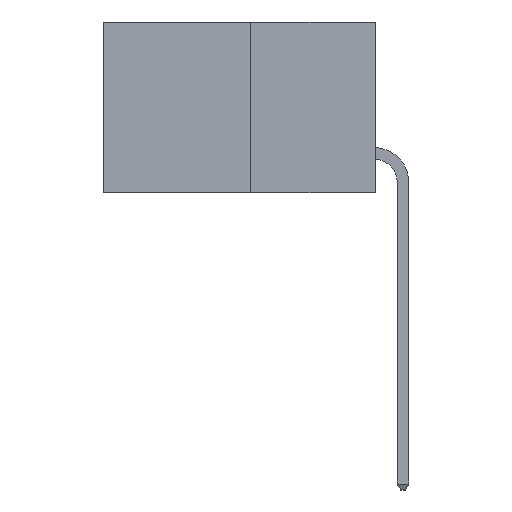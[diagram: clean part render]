
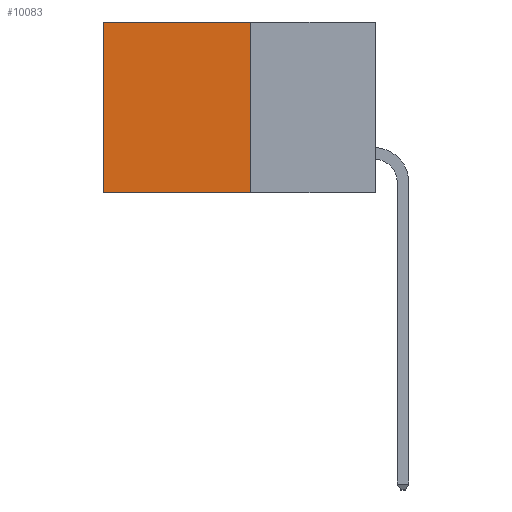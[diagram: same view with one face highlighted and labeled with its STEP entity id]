
A CAD part, left-side view. The second image highlights one B-rep face of the part: STEP entity #10083.
In plain terms, the highlighted planar face has unit normal (-1, 0, 0).
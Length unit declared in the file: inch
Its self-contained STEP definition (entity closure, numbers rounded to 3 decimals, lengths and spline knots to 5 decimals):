
#77 = CARTESIAN_POINT ( 'NONE',  ( 0.277, 0.27, -0.37 ) ) ;
#220 = VECTOR ( 'NONE', #15139, 39.37008 ) ;
#687 = LINE ( 'NONE', #77, #1678 ) ;
#996 = DIRECTION ( 'NONE',  ( 0., 1., 0. ) ) ;
#1178 = DIRECTION ( 'NONE',  ( 1., 0., 0. ) ) ;
#1315 = CARTESIAN_POINT ( 'NONE',  ( 0.277, 0.27, -0.37 ) ) ;
#1673 = DIRECTION ( 'NONE',  ( 0., 0., -1. ) ) ;
#1678 = VECTOR ( 'NONE', #1673, 39.37008 ) ;
#2572 = CARTESIAN_POINT ( 'NONE',  ( 0.277, 0.27, -0.37 ) ) ;
#3285 = VERTEX_POINT ( 'NONE', #3887 ) ;
#3887 = CARTESIAN_POINT ( 'NONE',  ( 0.277, 0.27, 0. ) ) ;
#4393 = CARTESIAN_POINT ( 'NONE',  ( 0.277, 0.27, 0. ) ) ;
#4779 = AXIS2_PLACEMENT_3D ( 'NONE', #8943, #1178, #11983 ) ;
#5387 = VERTEX_POINT ( 'NONE', #1315 ) ;
#6457 = ORIENTED_EDGE ( 'NONE', *, *, #10498, .T. ) ;
#6801 = CARTESIAN_POINT ( 'NONE',  ( 0.277, 0.59, 0. ) ) ;
#6888 = DIRECTION ( 'NONE',  ( 0., 0., -1. ) ) ;
#7182 = ORIENTED_EDGE ( 'NONE', *, *, #16518, .F. ) ;
#8208 = VECTOR ( 'NONE', #6888, 39.37008 ) ;
#8545 = LINE ( 'NONE', #4393, #220 ) ;
#8703 = LINE ( 'NONE', #12961, #8208 ) ;
#8943 = CARTESIAN_POINT ( 'NONE',  ( 0.277, 0.27, -0.37 ) ) ;
#9246 = ORIENTED_EDGE ( 'NONE', *, *, #15953, .T. ) ;
#10083 = ADVANCED_FACE ( 'NONE', ( #12252 ), #18022, .F. ) ;
#10480 = CARTESIAN_POINT ( 'NONE',  ( 0.277, 0.59, -0.37 ) ) ;
#10498 = EDGE_CURVE ( 'NONE', #16327, #15266, #8703, .T. ) ;
#11983 = DIRECTION ( 'NONE',  ( 0., 0., -1. ) ) ;
#12252 = FACE_OUTER_BOUND ( 'NONE', #18835, .T. ) ;
#12961 = CARTESIAN_POINT ( 'NONE',  ( 0.277, 0.59, -0.37 ) ) ;
#14202 = LINE ( 'NONE', #2572, #17777 ) ;
#15139 = DIRECTION ( 'NONE',  ( 0., 1., 0. ) ) ;
#15266 = VERTEX_POINT ( 'NONE', #10480 ) ;
#15953 = EDGE_CURVE ( 'NONE', #3285, #16327, #8545, .T. ) ;
#16229 = ORIENTED_EDGE ( 'NONE', *, *, #16783, .F. ) ;
#16327 = VERTEX_POINT ( 'NONE', #6801 ) ;
#16518 = EDGE_CURVE ( 'NONE', #5387, #15266, #14202, .T. ) ;
#16783 = EDGE_CURVE ( 'NONE', #3285, #5387, #687, .T. ) ;
#17777 = VECTOR ( 'NONE', #996, 39.37008 ) ;
#18022 = PLANE ( 'NONE',  #4779 ) ;
#18835 = EDGE_LOOP ( 'NONE', ( #6457, #7182, #16229, #9246 ) ) ;
